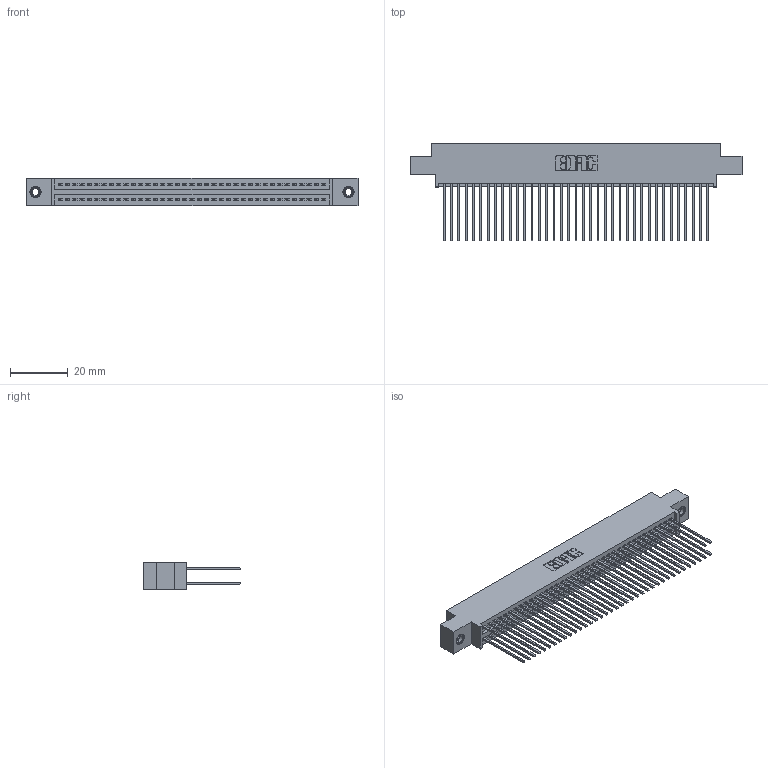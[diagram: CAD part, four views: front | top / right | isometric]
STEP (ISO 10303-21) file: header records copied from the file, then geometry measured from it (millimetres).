
FILE_DESCRIPTION (( 'STEP AP203' ), '1' );
FILE_NAME ('345-074-541-808.STEP', '2018-10-02T12:33:54', ( '' ), ( '' ), 'SwSTEP 2.0', 'SolidWorks 2016', '' );
FILE_SCHEMA (( 'CONFIG_CONTROL_DESIGN' ));
Length unit declared in the file: inch
Products named in the file (4): 345 Part_0.170 Offset - 0.156 Dia-TI; 345-292-001_345-293-141; 345-074-541-808; 345-250-001_345-250-003-102
Assembly tree (77 placements, depth 2):
  345-074-541-808
    345 Part_0.170 Offset - 0.156 Dia-TI
    345-292-001_345-293-141  x74
    345-250-001_345-250-003-102  x2
Bounding box: 115.19 x 33.96 x 9.4 mm (x, y, z)
Volume: 11447.8 mm3; surface area: 18977.6 mm2
Topology: 77 solids, 77 shells, 3890 faces, 11515 edges, 7570 vertices
Faces by surface type: plane 2558, cylinder 1316, cone 12, torus 4
Entity records: 31040 total; most frequent: CARTESIAN_POINT 5191, ORIENTED_EDGE 5118, DIRECTION 4609, EDGE_CURVE 2559, VECTOR 2259, LINE 2259, VERTEX_POINT 1700, AXIS2_PLACEMENT_3D 1175
